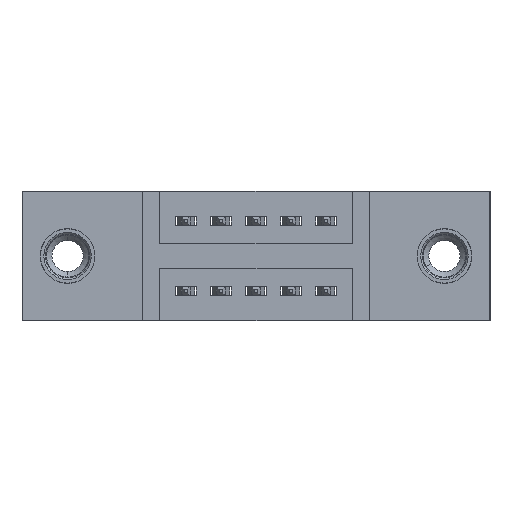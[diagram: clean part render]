
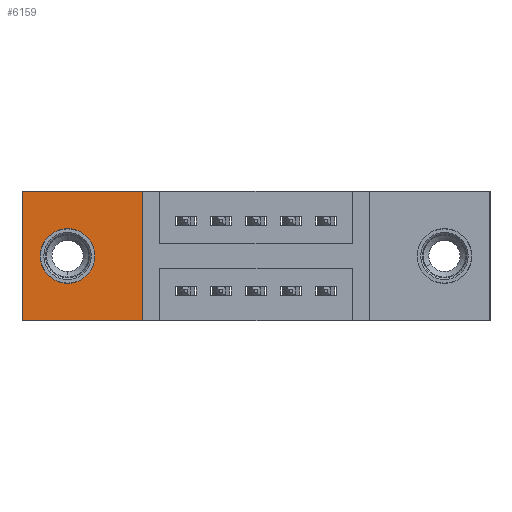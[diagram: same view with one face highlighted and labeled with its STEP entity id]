
A CAD part, front view. The second image highlights one B-rep face of the part: STEP entity #6159.
In plain terms, the highlighted planar face has unit normal (0, -1, 0).
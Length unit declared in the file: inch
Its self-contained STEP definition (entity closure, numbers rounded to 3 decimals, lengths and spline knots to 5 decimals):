
#253 = DIRECTION ( 'NONE',  ( 0., -1., 0. ) ) ;
#336 = FACE_OUTER_BOUND ( 'NONE', #6289, .T. ) ;
#676 = VECTOR ( 'NONE', #4804, 39.37008 ) ;
#679 = CARTESIAN_POINT ( 'NONE',  ( 0., 0.11, 0. ) ) ;
#683 = CARTESIAN_POINT ( 'NONE',  ( 0., 0.11, -0.37 ) ) ;
#996 = LINE ( 'NONE', #6317, #2671 ) ;
#1538 = EDGE_CURVE ( 'NONE', #3390, #9968, #996, .T. ) ;
#1931 = LINE ( 'NONE', #683, #676 ) ;
#2006 = VERTEX_POINT ( 'NONE', #4005 ) ;
#2058 = DIRECTION ( 'NONE',  ( 0., 0., 1. ) ) ;
#2111 = VERTEX_POINT ( 'NONE', #9050 ) ;
#2622 = CARTESIAN_POINT ( 'NONE',  ( 0., 0.11, -0.37 ) ) ;
#2671 = VECTOR ( 'NONE', #4261, 39.37008 ) ;
#3346 = FACE_BOUND ( 'NONE', #5679, .T. ) ;
#3390 = VERTEX_POINT ( 'NONE', #4151 ) ;
#3796 = DIRECTION ( 'NONE',  ( 0., 0., -1. ) ) ;
#4005 = CARTESIAN_POINT ( 'NONE',  ( 0.13, 0.11, -0.263 ) ) ;
#4123 = EDGE_CURVE ( 'NONE', #6091, #2006, #8700, .T. ) ;
#4151 = CARTESIAN_POINT ( 'NONE',  ( 0.3425, 0.11, 0. ) ) ;
#4261 = DIRECTION ( 'NONE',  ( -1., 0., 0. ) ) ;
#4541 = CARTESIAN_POINT ( 'NONE',  ( 0.3425, 0.11, 0. ) ) ;
#4566 = DIRECTION ( 'NONE',  ( 0., 0., -1. ) ) ;
#4663 = AXIS2_PLACEMENT_3D ( 'NONE', #5704, #253, #8913 ) ;
#4804 = DIRECTION ( 'NONE',  ( 1., 0., 0. ) ) ;
#4822 = ORIENTED_EDGE ( 'NONE', *, *, #8238, .F. ) ;
#5277 = VECTOR ( 'NONE', #2058, 39.37008 ) ;
#5367 = CARTESIAN_POINT ( 'NONE',  ( 0., 0.11, 0. ) ) ;
#5679 = EDGE_LOOP ( 'NONE', ( #8273, #4822 ) ) ;
#5704 = CARTESIAN_POINT ( 'NONE',  ( 0., 0.11, -0.37 ) ) ;
#6020 = ORIENTED_EDGE ( 'NONE', *, *, #1538, .T. ) ;
#6091 = VERTEX_POINT ( 'NONE', #9109 ) ;
#6146 = ORIENTED_EDGE ( 'NONE', *, *, #7602, .T. ) ;
#6152 = CARTESIAN_POINT ( 'NONE',  ( 0.13, 0.11, -0.185 ) ) ;
#6159 = ADVANCED_FACE ( 'NONE', ( #3346, #336 ), #7388, .T. ) ;
#6289 = EDGE_LOOP ( 'NONE', ( #7187, #6146, #9529, #6020 ) ) ;
#6317 = CARTESIAN_POINT ( 'NONE',  ( 0., 0.11, 0. ) ) ;
#6930 = DIRECTION ( 'NONE',  ( 0., -1., 0. ) ) ;
#6946 = DIRECTION ( 'NONE',  ( 0., -1., 0. ) ) ;
#7187 = ORIENTED_EDGE ( 'NONE', *, *, #9940, .T. ) ;
#7388 = PLANE ( 'NONE',  #4663 ) ;
#7602 = EDGE_CURVE ( 'NONE', #10164, #2111, #1931, .T. ) ;
#7757 = DIRECTION ( 'NONE',  ( 0., 0., -1. ) ) ;
#7812 = AXIS2_PLACEMENT_3D ( 'NONE', #10194, #6946, #7757 ) ;
#7953 = EDGE_CURVE ( 'NONE', #2111, #3390, #9340, .T. ) ;
#8238 = EDGE_CURVE ( 'NONE', #2006, #6091, #9931, .T. ) ;
#8273 = ORIENTED_EDGE ( 'NONE', *, *, #4123, .F. ) ;
#8447 = AXIS2_PLACEMENT_3D ( 'NONE', #6152, #6930, #4566 ) ;
#8643 = VECTOR ( 'NONE', #3796, 39.37008 ) ;
#8700 = CIRCLE ( 'NONE', #7812, 0.078 ) ;
#8893 = LINE ( 'NONE', #5367, #8643 ) ;
#8913 = DIRECTION ( 'NONE',  ( 0., 0., -1. ) ) ;
#9050 = CARTESIAN_POINT ( 'NONE',  ( 0.3425, 0.11, -0.37 ) ) ;
#9109 = CARTESIAN_POINT ( 'NONE',  ( 0.13, 0.11, -0.107 ) ) ;
#9340 = LINE ( 'NONE', #4541, #5277 ) ;
#9529 = ORIENTED_EDGE ( 'NONE', *, *, #7953, .T. ) ;
#9931 = CIRCLE ( 'NONE', #8447, 0.078 ) ;
#9940 = EDGE_CURVE ( 'NONE', #9968, #10164, #8893, .T. ) ;
#9968 = VERTEX_POINT ( 'NONE', #679 ) ;
#10164 = VERTEX_POINT ( 'NONE', #2622 ) ;
#10194 = CARTESIAN_POINT ( 'NONE',  ( 0.13, 0.11, -0.185 ) ) ;
